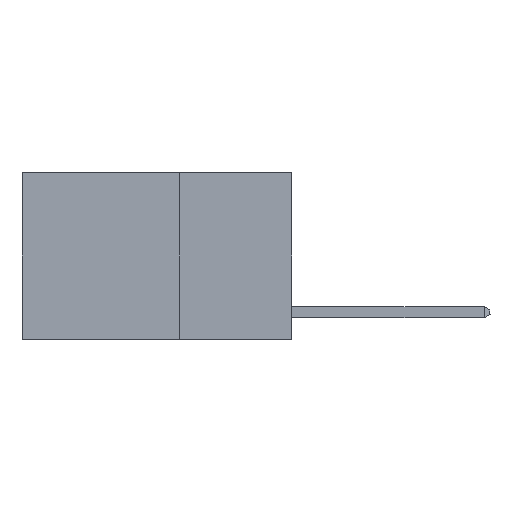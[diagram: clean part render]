
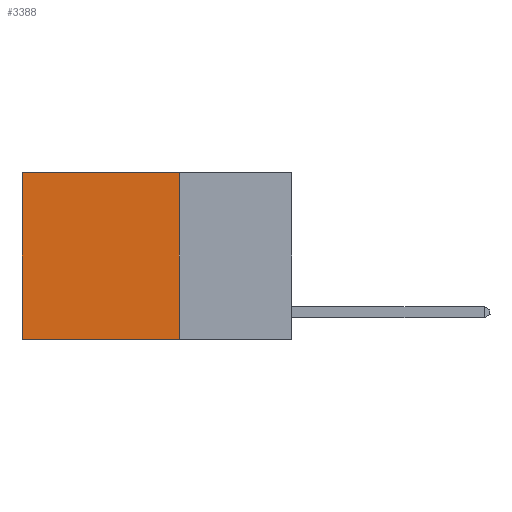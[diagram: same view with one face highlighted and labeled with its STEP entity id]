
A CAD part, left-side view. The second image highlights one B-rep face of the part: STEP entity #3388.
In plain terms, the highlighted planar face has unit normal (-1, 0, 0).
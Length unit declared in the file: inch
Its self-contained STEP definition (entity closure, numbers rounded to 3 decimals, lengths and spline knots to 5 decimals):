
#818 = CARTESIAN_POINT ( 'NONE',  ( 0.2625, 0.6, 0. ) ) ;
#1337 = CARTESIAN_POINT ( 'NONE',  ( 0.2625, 0.25, -0.37 ) ) ;
#1671 = DIRECTION ( 'NONE',  ( 0., 0., -1. ) ) ;
#1790 = CARTESIAN_POINT ( 'NONE',  ( 0.2625, 0.25, 0. ) ) ;
#1900 = EDGE_CURVE ( 'NONE', #4241, #7259, #4574, .T. ) ;
#1910 = EDGE_CURVE ( 'NONE', #4241, #8445, #9957, .T. ) ;
#2141 = VECTOR ( 'NONE', #1671, 39.37008 ) ;
#2547 = DIRECTION ( 'NONE',  ( 0., 0., -1. ) ) ;
#3001 = LINE ( 'NONE', #5260, #6551 ) ;
#3103 = DIRECTION ( 'NONE',  ( 0., 1., 0. ) ) ;
#3150 = CARTESIAN_POINT ( 'NONE',  ( 0.2625, 0.25, 0. ) ) ;
#3289 = VECTOR ( 'NONE', #6871, 39.37008 ) ;
#3388 = ADVANCED_FACE ( 'NONE', ( #5210 ), #7850, .F. ) ;
#3744 = VECTOR ( 'NONE', #9232, 39.37008 ) ;
#4205 = ORIENTED_EDGE ( 'NONE', *, *, #9260, .T. ) ;
#4241 = VERTEX_POINT ( 'NONE', #9978 ) ;
#4574 = LINE ( 'NONE', #7587, #3744 ) ;
#5059 = EDGE_CURVE ( 'NONE', #7259, #5318, #3001, .T. ) ;
#5210 = FACE_OUTER_BOUND ( 'NONE', #8177, .T. ) ;
#5260 = CARTESIAN_POINT ( 'NONE',  ( 0.2625, 0.25, -0.37 ) ) ;
#5318 = VERTEX_POINT ( 'NONE', #5774 ) ;
#5765 = AXIS2_PLACEMENT_3D ( 'NONE', #1790, #9436, #2547 ) ;
#5774 = CARTESIAN_POINT ( 'NONE',  ( 0.2625, 0.6, -0.37 ) ) ;
#5806 = ORIENTED_EDGE ( 'NONE', *, *, #1900, .F. ) ;
#6551 = VECTOR ( 'NONE', #3103, 39.37008 ) ;
#6871 = DIRECTION ( 'NONE',  ( 0., 1., 0. ) ) ;
#7259 = VERTEX_POINT ( 'NONE', #1337 ) ;
#7587 = CARTESIAN_POINT ( 'NONE',  ( 0.2625, 0.25, 0. ) ) ;
#7708 = ORIENTED_EDGE ( 'NONE', *, *, #1910, .T. ) ;
#7850 = PLANE ( 'NONE',  #5765 ) ;
#8177 = EDGE_LOOP ( 'NONE', ( #4205, #8520, #5806, #7708 ) ) ;
#8445 = VERTEX_POINT ( 'NONE', #9607 ) ;
#8520 = ORIENTED_EDGE ( 'NONE', *, *, #5059, .F. ) ;
#8721 = LINE ( 'NONE', #818, #2141 ) ;
#9232 = DIRECTION ( 'NONE',  ( 0., 0., -1. ) ) ;
#9260 = EDGE_CURVE ( 'NONE', #8445, #5318, #8721, .T. ) ;
#9436 = DIRECTION ( 'NONE',  ( 1., 0., 0. ) ) ;
#9607 = CARTESIAN_POINT ( 'NONE',  ( 0.2625, 0.6, 0. ) ) ;
#9957 = LINE ( 'NONE', #3150, #3289 ) ;
#9978 = CARTESIAN_POINT ( 'NONE',  ( 0.2625, 0.25, 0. ) ) ;
